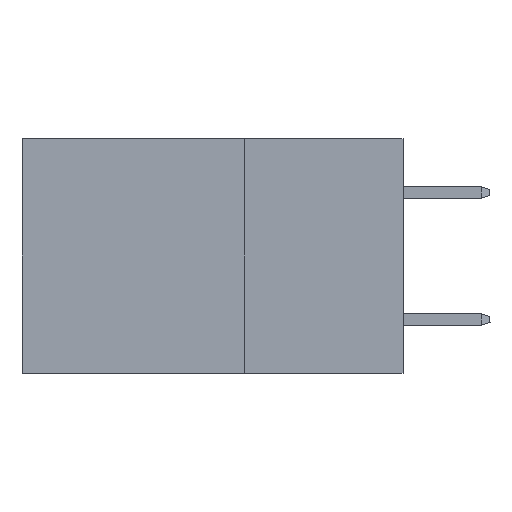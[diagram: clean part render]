
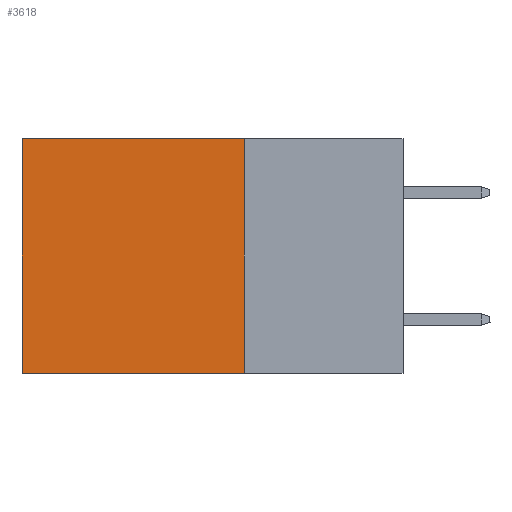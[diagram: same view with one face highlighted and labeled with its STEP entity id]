
A CAD part, left-side view. The second image highlights one B-rep face of the part: STEP entity #3618.
In plain terms, the highlighted planar face has unit normal (-1, 0, 0).
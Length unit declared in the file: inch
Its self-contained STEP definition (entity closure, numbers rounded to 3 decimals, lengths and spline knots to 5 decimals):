
#177 = ORIENTED_EDGE ( 'NONE', *, *, #26687, .F. ) ;
#831 = PLANE ( 'NONE',  #21927 ) ;
#1883 = LINE ( 'NONE', #10137, #24514 ) ;
#2477 = EDGE_CURVE ( 'NONE', #22074, #26171, #1883, .T. ) ;
#2906 = FACE_OUTER_BOUND ( 'NONE', #13312, .T. ) ;
#3178 = VECTOR ( 'NONE', #5612, 39.37008 ) ;
#3393 = DIRECTION ( 'NONE',  ( 0., 0., -1. ) ) ;
#3618 = ADVANCED_FACE ( 'NONE', ( #2906 ), #831, .F. ) ;
#4073 = ORIENTED_EDGE ( 'NONE', *, *, #11590, .T. ) ;
#5190 = CARTESIAN_POINT ( 'NONE',  ( 0.2875, 0.6, 0. ) ) ;
#5612 = DIRECTION ( 'NONE',  ( 0., 1., 0. ) ) ;
#6838 = LINE ( 'NONE', #5190, #17791 ) ;
#7000 = VERTEX_POINT ( 'NONE', #20506 ) ;
#7042 = CARTESIAN_POINT ( 'NONE',  ( 0.2875, 0.25, 0. ) ) ;
#7809 = EDGE_CURVE ( 'NONE', #23581, #7000, #6838, .T. ) ;
#8701 = LINE ( 'NONE', #7042, #25164 ) ;
#9254 = ORIENTED_EDGE ( 'NONE', *, *, #7809, .T. ) ;
#9609 = CARTESIAN_POINT ( 'NONE',  ( 0.2875, 0.25, -0.37 ) ) ;
#10137 = CARTESIAN_POINT ( 'NONE',  ( 0.2875, 0.25, 0. ) ) ;
#11152 = DIRECTION ( 'NONE',  ( 1., 0., 0. ) ) ;
#11165 = DIRECTION ( 'NONE',  ( 0., 1., 0. ) ) ;
#11590 = EDGE_CURVE ( 'NONE', #22074, #23581, #8701, .T. ) ;
#13312 = EDGE_LOOP ( 'NONE', ( #9254, #177, #24121, #4073 ) ) ;
#15414 = CARTESIAN_POINT ( 'NONE',  ( 0.2875, 0.25, -0.37 ) ) ;
#17791 = VECTOR ( 'NONE', #3393, 39.37008 ) ;
#18121 = LINE ( 'NONE', #9609, #3178 ) ;
#19211 = CARTESIAN_POINT ( 'NONE',  ( 0.2875, 0.25, 0. ) ) ;
#20506 = CARTESIAN_POINT ( 'NONE',  ( 0.2875, 0.6, -0.37 ) ) ;
#21887 = DIRECTION ( 'NONE',  ( 0., 0., -1. ) ) ;
#21927 = AXIS2_PLACEMENT_3D ( 'NONE', #23946, #11152, #21887 ) ;
#22074 = VERTEX_POINT ( 'NONE', #19211 ) ;
#23581 = VERTEX_POINT ( 'NONE', #24433 ) ;
#23946 = CARTESIAN_POINT ( 'NONE',  ( 0.2875, 0.25, 0. ) ) ;
#24121 = ORIENTED_EDGE ( 'NONE', *, *, #2477, .F. ) ;
#24433 = CARTESIAN_POINT ( 'NONE',  ( 0.2875, 0.6, 0. ) ) ;
#24514 = VECTOR ( 'NONE', #24725, 39.37008 ) ;
#24725 = DIRECTION ( 'NONE',  ( 0., 0., -1. ) ) ;
#25164 = VECTOR ( 'NONE', #11165, 39.37008 ) ;
#26171 = VERTEX_POINT ( 'NONE', #15414 ) ;
#26687 = EDGE_CURVE ( 'NONE', #26171, #7000, #18121, .T. ) ;
